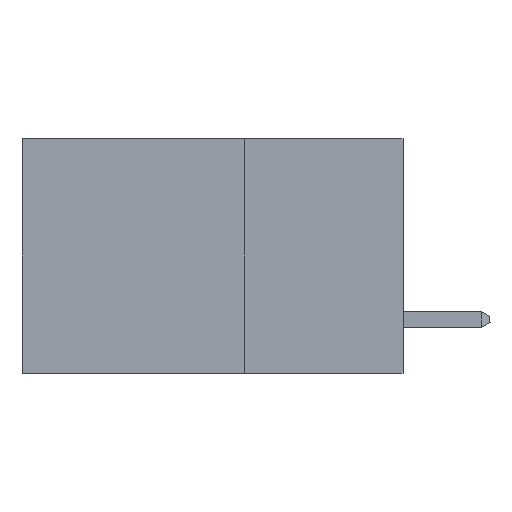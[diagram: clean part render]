
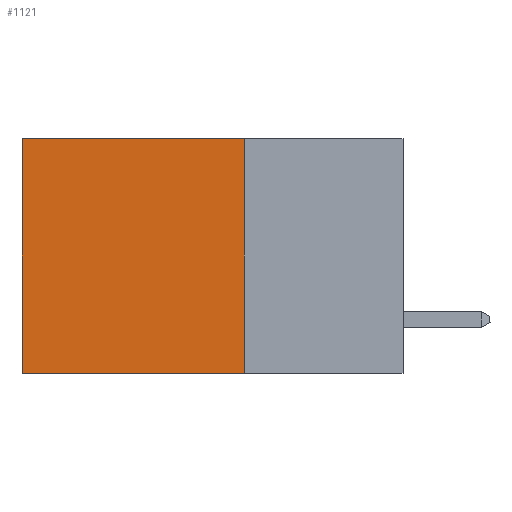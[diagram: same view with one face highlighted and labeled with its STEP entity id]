
A CAD part, left-side view. The second image highlights one B-rep face of the part: STEP entity #1121.
In plain terms, the highlighted planar face has unit normal (-1, 0, 0).
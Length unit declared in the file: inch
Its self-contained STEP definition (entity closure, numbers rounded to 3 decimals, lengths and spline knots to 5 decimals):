
#1121 = ADVANCED_FACE ( 'NONE', ( #41526 ), #27378, .F. ) ;
#1513 = LINE ( 'NONE', #11399, #2537 ) ;
#2138 = CARTESIAN_POINT ( 'NONE',  ( 0.2875, 0.25, -0.37 ) ) ;
#2298 = DIRECTION ( 'NONE',  ( 0., 1., 0. ) ) ;
#2537 = VECTOR ( 'NONE', #11970, 39.37008 ) ;
#3620 = EDGE_CURVE ( 'NONE', #33459, #6333, #1513, .T. ) ;
#4500 = ORIENTED_EDGE ( 'NONE', *, *, #3620, .F. ) ;
#4920 = VERTEX_POINT ( 'NONE', #15416 ) ;
#5047 = ORIENTED_EDGE ( 'NONE', *, *, #17066, .F. ) ;
#6333 = VERTEX_POINT ( 'NONE', #26438 ) ;
#7703 = ORIENTED_EDGE ( 'NONE', *, *, #10442, .T. ) ;
#8026 = DIRECTION ( 'NONE',  ( 0., 0., -1. ) ) ;
#8752 = CARTESIAN_POINT ( 'NONE',  ( 0.2875, 0.25, 0. ) ) ;
#9367 = CARTESIAN_POINT ( 'NONE',  ( 0.2875, 0.6, 0. ) ) ;
#10442 = EDGE_CURVE ( 'NONE', #25006, #4920, #33724, .T. ) ;
#11034 = CARTESIAN_POINT ( 'NONE',  ( 0.2875, 0.25, 0. ) ) ;
#11399 = CARTESIAN_POINT ( 'NONE',  ( 0.2875, 0.25, 0. ) ) ;
#11830 = DIRECTION ( 'NONE',  ( 0., 1., 0. ) ) ;
#11970 = DIRECTION ( 'NONE',  ( 0., 0., -1. ) ) ;
#14128 = EDGE_CURVE ( 'NONE', #33459, #25006, #23823, .T. ) ;
#15416 = CARTESIAN_POINT ( 'NONE',  ( 0.2875, 0.6, -0.37 ) ) ;
#15691 = ORIENTED_EDGE ( 'NONE', *, *, #14128, .T. ) ;
#17066 = EDGE_CURVE ( 'NONE', #6333, #4920, #32035, .T. ) ;
#20661 = EDGE_LOOP ( 'NONE', ( #7703, #5047, #4500, #15691 ) ) ;
#23745 = VECTOR ( 'NONE', #8026, 39.37008 ) ;
#23823 = LINE ( 'NONE', #8752, #32775 ) ;
#24566 = DIRECTION ( 'NONE',  ( 1., 0., 0. ) ) ;
#24864 = DIRECTION ( 'NONE',  ( 0., 0., -1. ) ) ;
#25006 = VERTEX_POINT ( 'NONE', #39840 ) ;
#26438 = CARTESIAN_POINT ( 'NONE',  ( 0.2875, 0.25, -0.37 ) ) ;
#26755 = AXIS2_PLACEMENT_3D ( 'NONE', #31349, #24566, #24864 ) ;
#27378 = PLANE ( 'NONE',  #26755 ) ;
#30977 = VECTOR ( 'NONE', #11830, 39.37008 ) ;
#31349 = CARTESIAN_POINT ( 'NONE',  ( 0.2875, 0.25, 0. ) ) ;
#32035 = LINE ( 'NONE', #2138, #30977 ) ;
#32775 = VECTOR ( 'NONE', #2298, 39.37008 ) ;
#33459 = VERTEX_POINT ( 'NONE', #11034 ) ;
#33724 = LINE ( 'NONE', #9367, #23745 ) ;
#39840 = CARTESIAN_POINT ( 'NONE',  ( 0.2875, 0.6, 0. ) ) ;
#41526 = FACE_OUTER_BOUND ( 'NONE', #20661, .T. ) ;
